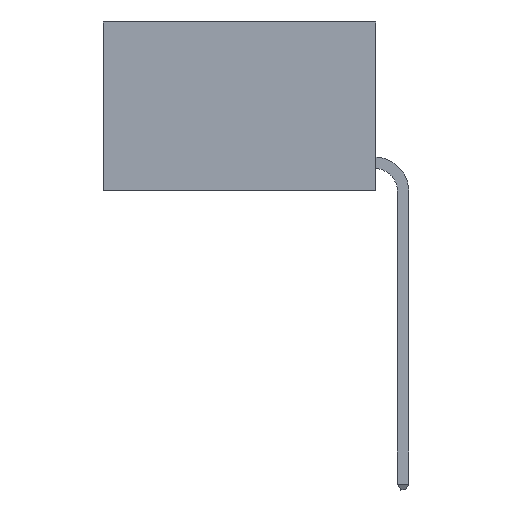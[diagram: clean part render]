
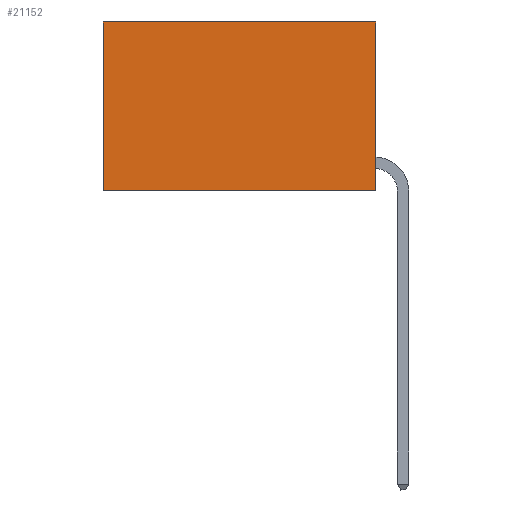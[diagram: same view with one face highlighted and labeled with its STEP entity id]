
A CAD part, left-side view. The second image highlights one B-rep face of the part: STEP entity #21152.
In plain terms, the highlighted planar face has unit normal (-1, 0, 0).
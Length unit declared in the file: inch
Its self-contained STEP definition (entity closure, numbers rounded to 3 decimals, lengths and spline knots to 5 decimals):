
#263 = CARTESIAN_POINT ( 'NONE',  ( 0.2625, 0.6, -0.37 ) ) ;
#604 = ORIENTED_EDGE ( 'NONE', *, *, #14034, .F. ) ;
#1091 = CARTESIAN_POINT ( 'NONE',  ( 0.2625, 0.6, 0. ) ) ;
#2099 = EDGE_CURVE ( 'NONE', #7926, #16956, #16787, .T. ) ;
#2751 = DIRECTION ( 'NONE',  ( 0., 0., -1. ) ) ;
#2918 = ORIENTED_EDGE ( 'NONE', *, *, #2099, .T. ) ;
#3717 = CARTESIAN_POINT ( 'NONE',  ( 0.2625, 0., 0. ) ) ;
#4057 = VECTOR ( 'NONE', #2751, 39.37008 ) ;
#4068 = ORIENTED_EDGE ( 'NONE', *, *, #20025, .T. ) ;
#4940 = EDGE_CURVE ( 'NONE', #15297, #20412, #22445, .T. ) ;
#5183 = VECTOR ( 'NONE', #10970, 39.37008 ) ;
#5352 = CARTESIAN_POINT ( 'NONE',  ( 0.2625, 0., 0. ) ) ;
#5443 = EDGE_LOOP ( 'NONE', ( #4068, #10669, #604, #2918 ) ) ;
#6486 = CARTESIAN_POINT ( 'NONE',  ( 0.2625, 0., 0. ) ) ;
#6886 = FACE_OUTER_BOUND ( 'NONE', #5443, .T. ) ;
#7714 = VECTOR ( 'NONE', #11233, 39.37008 ) ;
#7926 = VERTEX_POINT ( 'NONE', #5352 ) ;
#10179 = VECTOR ( 'NONE', #24398, 39.37008 ) ;
#10669 = ORIENTED_EDGE ( 'NONE', *, *, #4940, .F. ) ;
#10970 = DIRECTION ( 'NONE',  ( 0., 1., 0. ) ) ;
#11233 = DIRECTION ( 'NONE',  ( 0., 1., 0. ) ) ;
#12181 = CARTESIAN_POINT ( 'NONE',  ( 0.2625, 0., -0.37 ) ) ;
#14034 = EDGE_CURVE ( 'NONE', #7926, #15297, #21424, .T. ) ;
#15289 = CARTESIAN_POINT ( 'NONE',  ( 0.2625, 0., -0.37 ) ) ;
#15297 = VERTEX_POINT ( 'NONE', #12181 ) ;
#16382 = PLANE ( 'NONE',  #18485 ) ;
#16787 = LINE ( 'NONE', #3717, #7714 ) ;
#16864 = CARTESIAN_POINT ( 'NONE',  ( 0.2625, 0.6, 0. ) ) ;
#16956 = VERTEX_POINT ( 'NONE', #1091 ) ;
#18473 = CARTESIAN_POINT ( 'NONE',  ( 0.2625, 0., 0. ) ) ;
#18485 = AXIS2_PLACEMENT_3D ( 'NONE', #18473, #22296, #20458 ) ;
#20025 = EDGE_CURVE ( 'NONE', #16956, #20412, #22670, .T. ) ;
#20412 = VERTEX_POINT ( 'NONE', #263 ) ;
#20458 = DIRECTION ( 'NONE',  ( 0., 0., -1. ) ) ;
#21152 = ADVANCED_FACE ( 'NONE', ( #6886 ), #16382, .F. ) ;
#21424 = LINE ( 'NONE', #6486, #4057 ) ;
#22296 = DIRECTION ( 'NONE',  ( 1., 0., 0. ) ) ;
#22445 = LINE ( 'NONE', #15289, #5183 ) ;
#22670 = LINE ( 'NONE', #16864, #10179 ) ;
#24398 = DIRECTION ( 'NONE',  ( 0., 0., -1. ) ) ;
